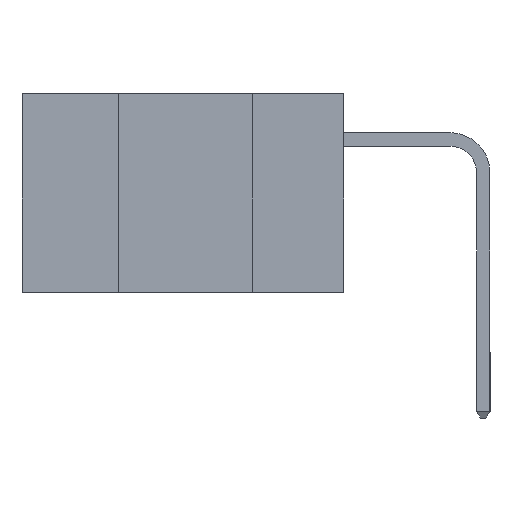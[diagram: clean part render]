
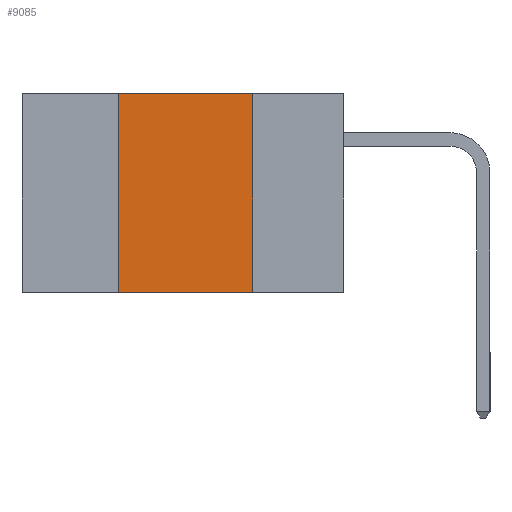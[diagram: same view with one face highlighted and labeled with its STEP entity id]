
A CAD part, left-side view. The second image highlights one B-rep face of the part: STEP entity #9085.
In plain terms, the highlighted planar face has unit normal (-1, 0, 0).
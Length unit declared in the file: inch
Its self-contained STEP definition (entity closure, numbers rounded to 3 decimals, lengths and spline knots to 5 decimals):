
#64 = VERTEX_POINT ( 'NONE', #14222 ) ;
#613 = ORIENTED_EDGE ( 'NONE', *, *, #2511, .T. ) ;
#1108 = CARTESIAN_POINT ( 'NONE',  ( 0., 0.17, 0. ) ) ;
#1386 = PLANE ( 'NONE',  #10704 ) ;
#1396 = VECTOR ( 'NONE', #7730, 39.37008 ) ;
#2511 = EDGE_CURVE ( 'NONE', #6418, #64, #6601, .T. ) ;
#3102 = LINE ( 'NONE', #1108, #1396 ) ;
#3346 = DIRECTION ( 'NONE',  ( 0., -1., 0. ) ) ;
#3459 = CARTESIAN_POINT ( 'NONE',  ( 0., 0.6, 0. ) ) ;
#3773 = LINE ( 'NONE', #3459, #9557 ) ;
#5096 = CARTESIAN_POINT ( 'NONE',  ( 0., 0.42, 0. ) ) ;
#5354 = CARTESIAN_POINT ( 'NONE',  ( 0., 0.42, 0. ) ) ;
#5616 = DIRECTION ( 'NONE',  ( 1., 0., 0. ) ) ;
#5653 = ORIENTED_EDGE ( 'NONE', *, *, #16944, .F. ) ;
#5830 = ORIENTED_EDGE ( 'NONE', *, *, #9567, .F. ) ;
#6418 = VERTEX_POINT ( 'NONE', #17642 ) ;
#6545 = VECTOR ( 'NONE', #13590, 39.37008 ) ;
#6601 = LINE ( 'NONE', #15032, #10684 ) ;
#7596 = VERTEX_POINT ( 'NONE', #5096 ) ;
#7730 = DIRECTION ( 'NONE',  ( 0., 0., -1. ) ) ;
#8045 = LINE ( 'NONE', #5354, #6545 ) ;
#8065 = DIRECTION ( 'NONE',  ( 0., -1., 0. ) ) ;
#8594 = ORIENTED_EDGE ( 'NONE', *, *, #8715, .F. ) ;
#8715 = EDGE_CURVE ( 'NONE', #7596, #10350, #3773, .T. ) ;
#9085 = ADVANCED_FACE ( 'NONE', ( #14358 ), #1386, .F. ) ;
#9557 = VECTOR ( 'NONE', #3346, 39.37008 ) ;
#9567 = EDGE_CURVE ( 'NONE', #6418, #7596, #8045, .T. ) ;
#10350 = VERTEX_POINT ( 'NONE', #16845 ) ;
#10684 = VECTOR ( 'NONE', #8065, 39.37008 ) ;
#10704 = AXIS2_PLACEMENT_3D ( 'NONE', #12507, #5616, #15468 ) ;
#12507 = CARTESIAN_POINT ( 'NONE',  ( 0., 0.6, 0. ) ) ;
#13590 = DIRECTION ( 'NONE',  ( 0., 0., 1. ) ) ;
#14222 = CARTESIAN_POINT ( 'NONE',  ( 0., 0.17, -0.37 ) ) ;
#14358 = FACE_OUTER_BOUND ( 'NONE', #16188, .T. ) ;
#15032 = CARTESIAN_POINT ( 'NONE',  ( 0., 0.6, -0.37 ) ) ;
#15468 = DIRECTION ( 'NONE',  ( 0., 0., -1. ) ) ;
#16188 = EDGE_LOOP ( 'NONE', ( #5653, #8594, #5830, #613 ) ) ;
#16845 = CARTESIAN_POINT ( 'NONE',  ( 0., 0.17, 0. ) ) ;
#16944 = EDGE_CURVE ( 'NONE', #10350, #64, #3102, .T. ) ;
#17642 = CARTESIAN_POINT ( 'NONE',  ( 0., 0.42, -0.37 ) ) ;
